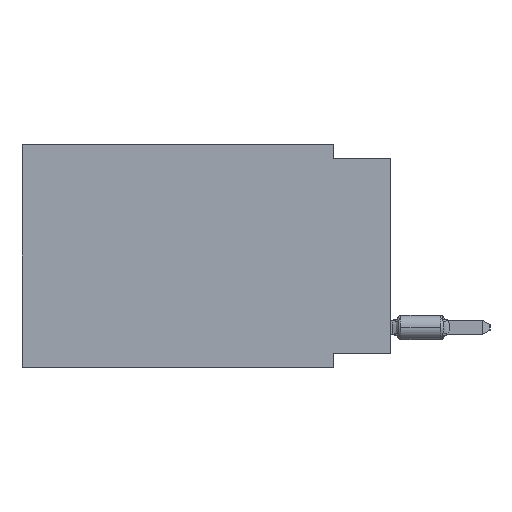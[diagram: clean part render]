
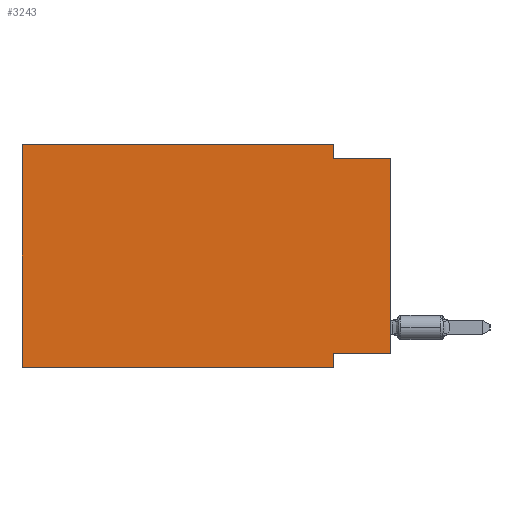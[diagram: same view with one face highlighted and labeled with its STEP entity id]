
A CAD part, left-side view. The second image highlights one B-rep face of the part: STEP entity #3243.
In plain terms, the highlighted planar face has unit normal (-1, 0, 0).
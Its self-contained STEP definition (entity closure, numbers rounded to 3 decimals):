
#6 = CARTESIAN_POINT ( 'NONE',  ( 0., 2.54, 0. ) ) ;
#264 = EDGE_CURVE ( 'NONE', #853, #39185, #30537, .T. ) ;
#320 = VERTEX_POINT ( 'NONE', #20877 ) ;
#853 = VERTEX_POINT ( 'NONE', #15770 ) ;
#2124 = CARTESIAN_POINT ( 'NONE',  ( 0., 16.383, 0. ) ) ;
#2591 = EDGE_CURVE ( 'NONE', #26722, #11237, #27129, .T. ) ;
#3243 = ADVANCED_FACE ( 'NONE', ( #16491 ), #29307, .F. ) ;
#3744 = DIRECTION ( 'NONE',  ( 0., -1., 0. ) ) ;
#4208 = CARTESIAN_POINT ( 'NONE',  ( 0., 0., 0. ) ) ;
#4242 = DIRECTION ( 'NONE',  ( 0., 0., -1. ) ) ;
#5760 = CARTESIAN_POINT ( 'NONE',  ( 0., 16.383, -9.906 ) ) ;
#5953 = VECTOR ( 'NONE', #12206, 1000. ) ;
#6211 = VECTOR ( 'NONE', #4242, 1000. ) ;
#8047 = DIRECTION ( 'NONE',  ( 0., 1., 0. ) ) ;
#8081 = CARTESIAN_POINT ( 'NONE',  ( 0., 0., -0.635 ) ) ;
#8093 = CARTESIAN_POINT ( 'NONE',  ( 0., 2.54, -9.906 ) ) ;
#8734 = ORIENTED_EDGE ( 'NONE', *, *, #264, .F. ) ;
#8789 = VECTOR ( 'NONE', #8047, 1000. ) ;
#9049 = DIRECTION ( 'NONE',  ( 0., -1., 0. ) ) ;
#9209 = ORIENTED_EDGE ( 'NONE', *, *, #24167, .F. ) ;
#9341 = EDGE_CURVE ( 'NONE', #320, #26722, #41004, .T. ) ;
#10122 = VECTOR ( 'NONE', #20381, 1000. ) ;
#10550 = EDGE_CURVE ( 'NONE', #13929, #41145, #34537, .T. ) ;
#11012 = VECTOR ( 'NONE', #40885, 1000. ) ;
#11068 = VECTOR ( 'NONE', #3744, 1000. ) ;
#11237 = VERTEX_POINT ( 'NONE', #18317 ) ;
#11323 = ORIENTED_EDGE ( 'NONE', *, *, #2591, .F. ) ;
#11972 = CARTESIAN_POINT ( 'NONE',  ( 0., 0., -0.635 ) ) ;
#12206 = DIRECTION ( 'NONE',  ( 0., 0., 1. ) ) ;
#13226 = VECTOR ( 'NONE', #9049, 1000. ) ;
#13929 = VERTEX_POINT ( 'NONE', #26428 ) ;
#14556 = CARTESIAN_POINT ( 'NONE',  ( 0., 2.54, -9.906 ) ) ;
#14790 = EDGE_CURVE ( 'NONE', #853, #24624, #30256, .T. ) ;
#15506 = ORIENTED_EDGE ( 'NONE', *, *, #31794, .F. ) ;
#15770 = CARTESIAN_POINT ( 'NONE',  ( 0., 0., -9.271 ) ) ;
#16297 = ORIENTED_EDGE ( 'NONE', *, *, #10550, .T. ) ;
#16491 = FACE_OUTER_BOUND ( 'NONE', #32860, .T. ) ;
#18317 = CARTESIAN_POINT ( 'NONE',  ( 0., 2.54, -0.635 ) ) ;
#20381 = DIRECTION ( 'NONE',  ( 0., 0., 1. ) ) ;
#20637 = CARTESIAN_POINT ( 'NONE',  ( 0., 2.54, 0. ) ) ;
#20877 = CARTESIAN_POINT ( 'NONE',  ( 0., 16.383, 0. ) ) ;
#20911 = DIRECTION ( 'NONE',  ( 0., -1., 0. ) ) ;
#21670 = CARTESIAN_POINT ( 'NONE',  ( 0., 16.383, 0. ) ) ;
#23479 = CARTESIAN_POINT ( 'NONE',  ( 0., 2.54, -9.271 ) ) ;
#24085 = LINE ( 'NONE', #8093, #11012 ) ;
#24167 = EDGE_CURVE ( 'NONE', #13929, #320, #25456, .T. ) ;
#24448 = AXIS2_PLACEMENT_3D ( 'NONE', #25522, #39168, #38970 ) ;
#24624 = VERTEX_POINT ( 'NONE', #11972 ) ;
#24715 = ORIENTED_EDGE ( 'NONE', *, *, #14790, .T. ) ;
#25456 = LINE ( 'NONE', #21670, #5953 ) ;
#25522 = CARTESIAN_POINT ( 'NONE',  ( 0., 16.383, 0. ) ) ;
#26428 = CARTESIAN_POINT ( 'NONE',  ( 0., 16.383, -9.906 ) ) ;
#26722 = VERTEX_POINT ( 'NONE', #6 ) ;
#27129 = LINE ( 'NONE', #20637, #6211 ) ;
#27424 = EDGE_CURVE ( 'NONE', #39185, #41145, #24085, .T. ) ;
#29307 = PLANE ( 'NONE',  #24448 ) ;
#30256 = LINE ( 'NONE', #4208, #10122 ) ;
#30537 = LINE ( 'NONE', #37668, #8789 ) ;
#31028 = ORIENTED_EDGE ( 'NONE', *, *, #9341, .F. ) ;
#31794 = EDGE_CURVE ( 'NONE', #11237, #24624, #37286, .T. ) ;
#32860 = EDGE_LOOP ( 'NONE', ( #24715, #15506, #11323, #31028, #9209, #16297, #36284, #8734 ) ) ;
#34537 = LINE ( 'NONE', #5760, #11068 ) ;
#36284 = ORIENTED_EDGE ( 'NONE', *, *, #27424, .F. ) ;
#37286 = LINE ( 'NONE', #8081, #41394 ) ;
#37668 = CARTESIAN_POINT ( 'NONE',  ( 0., 0., -9.271 ) ) ;
#38970 = DIRECTION ( 'NONE',  ( 0., 0., -1. ) ) ;
#39168 = DIRECTION ( 'NONE',  ( 1., 0., 0. ) ) ;
#39185 = VERTEX_POINT ( 'NONE', #23479 ) ;
#40885 = DIRECTION ( 'NONE',  ( 0., 0., -1. ) ) ;
#41004 = LINE ( 'NONE', #2124, #13226 ) ;
#41145 = VERTEX_POINT ( 'NONE', #14556 ) ;
#41394 = VECTOR ( 'NONE', #20911, 1000. ) ;
